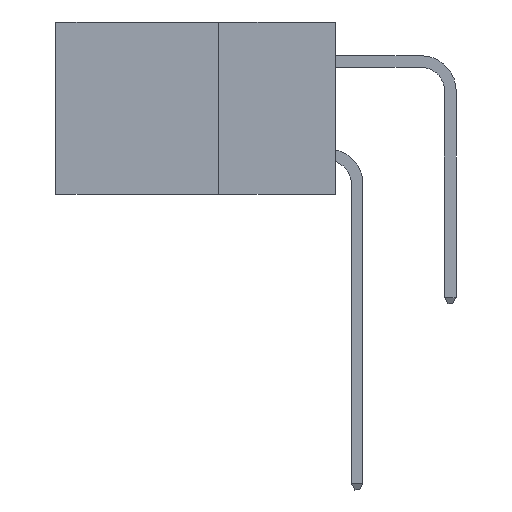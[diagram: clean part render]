
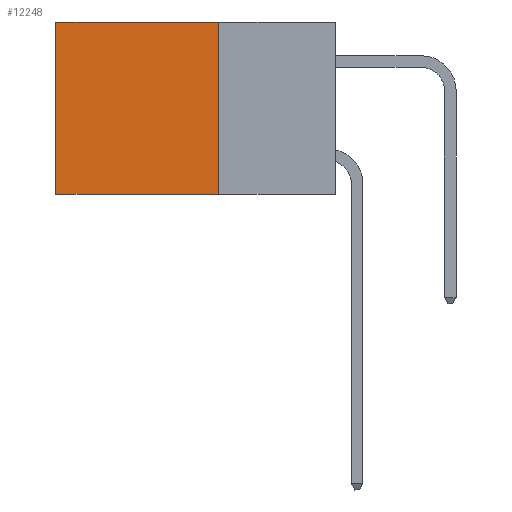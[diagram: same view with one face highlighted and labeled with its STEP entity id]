
A CAD part, left-side view. The second image highlights one B-rep face of the part: STEP entity #12248.
In plain terms, the highlighted planar face has unit normal (-1, 0, 0).
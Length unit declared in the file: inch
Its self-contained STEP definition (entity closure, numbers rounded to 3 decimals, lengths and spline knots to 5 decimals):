
#31 = DIRECTION ( 'NONE',  ( 0., 0., -1. ) ) ;
#497 = CARTESIAN_POINT ( 'NONE',  ( 0.2875, 0.6, 0. ) ) ;
#1153 = DIRECTION ( 'NONE',  ( 0., 0., -1. ) ) ;
#1175 = CARTESIAN_POINT ( 'NONE',  ( 0.2875, 0.25, 0. ) ) ;
#1478 = CARTESIAN_POINT ( 'NONE',  ( 0.2875, 0.6, -0.37 ) ) ;
#1693 = DIRECTION ( 'NONE',  ( 0., 0., -1. ) ) ;
#1895 = VERTEX_POINT ( 'NONE', #1478 ) ;
#2210 = ORIENTED_EDGE ( 'NONE', *, *, #12913, .F. ) ;
#2299 = LINE ( 'NONE', #6936, #8415 ) ;
#2393 = CARTESIAN_POINT ( 'NONE',  ( 0.2875, 0.25, 0. ) ) ;
#2950 = VERTEX_POINT ( 'NONE', #4883 ) ;
#3188 = EDGE_LOOP ( 'NONE', ( #9644, #7385, #2210, #7809 ) ) ;
#3865 = LINE ( 'NONE', #7252, #9902 ) ;
#4883 = CARTESIAN_POINT ( 'NONE',  ( 0.2875, 0.25, -0.37 ) ) ;
#5097 = CARTESIAN_POINT ( 'NONE',  ( 0.2875, 0.6, 0. ) ) ;
#5104 = VERTEX_POINT ( 'NONE', #2393 ) ;
#6094 = EDGE_CURVE ( 'NONE', #2950, #1895, #2299, .T. ) ;
#6098 = PLANE ( 'NONE',  #10311 ) ;
#6936 = CARTESIAN_POINT ( 'NONE',  ( 0.2875, 0.25, -0.37 ) ) ;
#7252 = CARTESIAN_POINT ( 'NONE',  ( 0.2875, 0.25, 0. ) ) ;
#7322 = DIRECTION ( 'NONE',  ( 1., 0., 0. ) ) ;
#7385 = ORIENTED_EDGE ( 'NONE', *, *, #6094, .F. ) ;
#7701 = FACE_OUTER_BOUND ( 'NONE', #3188, .T. ) ;
#7809 = ORIENTED_EDGE ( 'NONE', *, *, #9421, .T. ) ;
#8011 = VERTEX_POINT ( 'NONE', #5097 ) ;
#8052 = CARTESIAN_POINT ( 'NONE',  ( 0.2875, 0.25, 0. ) ) ;
#8415 = VECTOR ( 'NONE', #12938, 39.37008 ) ;
#8614 = VECTOR ( 'NONE', #1693, 39.37008 ) ;
#9371 = LINE ( 'NONE', #497, #8614 ) ;
#9421 = EDGE_CURVE ( 'NONE', #5104, #8011, #11159, .T. ) ;
#9644 = ORIENTED_EDGE ( 'NONE', *, *, #14093, .T. ) ;
#9902 = VECTOR ( 'NONE', #1153, 39.37008 ) ;
#10311 = AXIS2_PLACEMENT_3D ( 'NONE', #1175, #7322, #31 ) ;
#11159 = LINE ( 'NONE', #8052, #14005 ) ;
#12248 = ADVANCED_FACE ( 'NONE', ( #7701 ), #6098, .F. ) ;
#12835 = DIRECTION ( 'NONE',  ( 0., 1., 0. ) ) ;
#12913 = EDGE_CURVE ( 'NONE', #5104, #2950, #3865, .T. ) ;
#12938 = DIRECTION ( 'NONE',  ( 0., 1., 0. ) ) ;
#14005 = VECTOR ( 'NONE', #12835, 39.37008 ) ;
#14093 = EDGE_CURVE ( 'NONE', #8011, #1895, #9371, .T. ) ;
